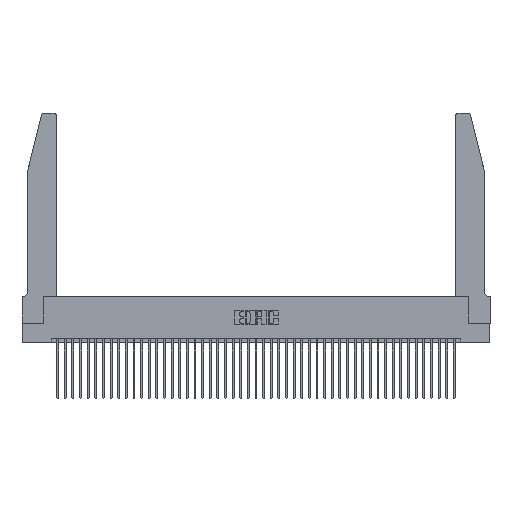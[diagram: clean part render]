
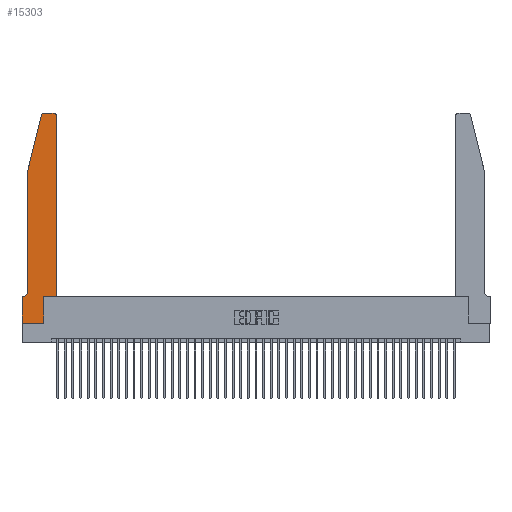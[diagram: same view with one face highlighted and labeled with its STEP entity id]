
A CAD part, top view. The second image highlights one B-rep face of the part: STEP entity #15303.
In plain terms, the highlighted planar face has unit normal (0, 0, 1).
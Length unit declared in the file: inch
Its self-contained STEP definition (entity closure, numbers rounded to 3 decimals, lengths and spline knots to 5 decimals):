
#76 = CARTESIAN_POINT ( 'NONE',  ( 0.0755, 0.35, 0.37 ) ) ;
#710 = DIRECTION ( 'NONE',  ( 1., 0., 0. ) ) ;
#795 = VERTEX_POINT ( 'NONE', #36567 ) ;
#1009 = CARTESIAN_POINT ( 'NONE',  ( 0., 0., 0.37 ) ) ;
#1309 = EDGE_CURVE ( 'NONE', #44725, #22038, #30585, .T. ) ;
#1569 = LINE ( 'NONE', #36733, #19284 ) ;
#1660 = DIRECTION ( 'NONE',  ( 0., 0., 1. ) ) ;
#2076 = VECTOR ( 'NONE', #38188, 39.37008 ) ;
#2180 = CIRCLE ( 'NONE', #6765, 0.07 ) ;
#2772 = VECTOR ( 'NONE', #710, 39.37008 ) ;
#3367 = DIRECTION ( 'NONE',  ( 0., 1., 0. ) ) ;
#3977 = AXIS2_PLACEMENT_3D ( 'NONE', #22750, #1660, #26181 ) ;
#4486 = EDGE_CURVE ( 'NONE', #9154, #10186, #36277, .T. ) ;
#6324 = DIRECTION ( 'NONE',  ( 0., 0., 1. ) ) ;
#6765 = AXIS2_PLACEMENT_3D ( 'NONE', #12347, #36340, #15891 ) ;
#7992 = ORIENTED_EDGE ( 'NONE', *, *, #33383, .T. ) ;
#8782 = EDGE_LOOP ( 'NONE', ( #35161, #17782, #32052, #16787, #7992, #31920, #22586, #39073, #15996, #11675, #17473, #20082 ) ) ;
#9097 = LINE ( 'NONE', #11024, #27553 ) ;
#9154 = VERTEX_POINT ( 'NONE', #36543 ) ;
#9280 = FACE_OUTER_BOUND ( 'NONE', #8782, .T. ) ;
#9546 = CARTESIAN_POINT ( 'NONE',  ( 0.0755, 2., 0.37 ) ) ;
#10186 = VERTEX_POINT ( 'NONE', #36451 ) ;
#11024 = CARTESIAN_POINT ( 'NONE',  ( 0.4505, 0.35, 0.37 ) ) ;
#11675 = ORIENTED_EDGE ( 'NONE', *, *, #24936, .T. ) ;
#12158 = EDGE_CURVE ( 'NONE', #10186, #16158, #44568, .T. ) ;
#12252 = CARTESIAN_POINT ( 'NONE',  ( 0.0755, 0.42, 0.37 ) ) ;
#12347 = CARTESIAN_POINT ( 'NONE',  ( 0.0055, 0.42, 0.37 ) ) ;
#13258 = LINE ( 'NONE', #28076, #21433 ) ;
#13936 = CARTESIAN_POINT ( 'NONE',  ( 0.2865, 0.35, 0.37 ) ) ;
#14322 = EDGE_CURVE ( 'NONE', #16159, #38533, #41130, .T. ) ;
#14345 = DIRECTION ( 'NONE',  ( 0., -1., 0. ) ) ;
#14538 = DIRECTION ( 'NONE',  ( 1., 0., 0. ) ) ;
#14761 = VERTEX_POINT ( 'NONE', #37540 ) ;
#15277 = DIRECTION ( 'NONE',  ( -0.239, -0.971, 0. ) ) ;
#15303 = ADVANCED_FACE ( 'NONE', ( #9280 ), #23843, .T. ) ;
#15891 = DIRECTION ( 'NONE',  ( -1., 0., 0. ) ) ;
#15937 = CARTESIAN_POINT ( 'NONE',  ( 0.0055, 0.35, 0.37 ) ) ;
#15996 = ORIENTED_EDGE ( 'NONE', *, *, #26676, .T. ) ;
#16158 = VERTEX_POINT ( 'NONE', #12252 ) ;
#16159 = VERTEX_POINT ( 'NONE', #15937 ) ;
#16787 = ORIENTED_EDGE ( 'NONE', *, *, #12158, .T. ) ;
#17473 = ORIENTED_EDGE ( 'NONE', *, *, #34103, .T. ) ;
#17782 = ORIENTED_EDGE ( 'NONE', *, *, #41490, .T. ) ;
#18174 = VECTOR ( 'NONE', #15277, 39.37008 ) ;
#19284 = VECTOR ( 'NONE', #40191, 39.37008 ) ;
#19387 = VERTEX_POINT ( 'NONE', #30235 ) ;
#20082 = ORIENTED_EDGE ( 'NONE', *, *, #31767, .T. ) ;
#20347 = CARTESIAN_POINT ( 'NONE',  ( 0.284, 2.72, 0.37 ) ) ;
#20458 = CARTESIAN_POINT ( 'NONE',  ( 0., 0., 0.37 ) ) ;
#20937 = EDGE_CURVE ( 'NONE', #38533, #44725, #39913, .T. ) ;
#21433 = VECTOR ( 'NONE', #34886, 39.37008 ) ;
#21814 = VECTOR ( 'NONE', #14345, 39.37008 ) ;
#22038 = VERTEX_POINT ( 'NONE', #27486 ) ;
#22586 = ORIENTED_EDGE ( 'NONE', *, *, #20937, .T. ) ;
#22750 = CARTESIAN_POINT ( 'NONE',  ( 0.4205, 2.72, 0.37 ) ) ;
#23774 = DIRECTION ( 'NONE',  ( 1., 0., 0. ) ) ;
#23843 = PLANE ( 'NONE',  #43394 ) ;
#24936 = EDGE_CURVE ( 'NONE', #40113, #19387, #9097, .T. ) ;
#26181 = DIRECTION ( 'NONE',  ( 1., 0., 0. ) ) ;
#26426 = VECTOR ( 'NONE', #37047, 39.37008 ) ;
#26676 = EDGE_CURVE ( 'NONE', #22038, #40113, #41310, .T. ) ;
#27154 = CARTESIAN_POINT ( 'NONE',  ( 0., 0.35, 0.37 ) ) ;
#27486 = CARTESIAN_POINT ( 'NONE',  ( 0.2865, 0., 0.37 ) ) ;
#27553 = VECTOR ( 'NONE', #14538, 39.37008 ) ;
#28076 = CARTESIAN_POINT ( 'NONE',  ( 0.2605, 2.75, 0.37 ) ) ;
#28304 = EDGE_CURVE ( 'NONE', #795, #14761, #13258, .T. ) ;
#28943 = CARTESIAN_POINT ( 'NONE',  ( 0.0755, 2., 0.37 ) ) ;
#30235 = CARTESIAN_POINT ( 'NONE',  ( 0.4505, 0.35, 0.37 ) ) ;
#30550 = DIRECTION ( 'NONE',  ( 1., 0., 0. ) ) ;
#30585 = LINE ( 'NONE', #1009, #2772 ) ;
#31767 = EDGE_CURVE ( 'NONE', #40876, #795, #31797, .T. ) ;
#31797 = CIRCLE ( 'NONE', #3977, 0.03 ) ;
#31920 = ORIENTED_EDGE ( 'NONE', *, *, #14322, .T. ) ;
#32052 = ORIENTED_EDGE ( 'NONE', *, *, #4486, .T. ) ;
#33383 = EDGE_CURVE ( 'NONE', #16158, #16159, #2180, .T. ) ;
#33966 = AXIS2_PLACEMENT_3D ( 'NONE', #20347, #44177, #23774 ) ;
#34103 = EDGE_CURVE ( 'NONE', #19387, #40876, #1569, .T. ) ;
#34222 = CARTESIAN_POINT ( 'NONE',  ( 0.4505, 2.72, 0.37 ) ) ;
#34863 = CARTESIAN_POINT ( 'NONE',  ( 0., 0., 0.37 ) ) ;
#34886 = DIRECTION ( 'NONE',  ( -1., 0., 0. ) ) ;
#35161 = ORIENTED_EDGE ( 'NONE', *, *, #28304, .T. ) ;
#36277 = LINE ( 'NONE', #28943, #18174 ) ;
#36340 = DIRECTION ( 'NONE',  ( 0., 0., -1. ) ) ;
#36451 = CARTESIAN_POINT ( 'NONE',  ( 0.0755, 2., 0.37 ) ) ;
#36543 = CARTESIAN_POINT ( 'NONE',  ( 0.25487, 2.72718, 0.37 ) ) ;
#36567 = CARTESIAN_POINT ( 'NONE',  ( 0.4205, 2.75, 0.37 ) ) ;
#36733 = CARTESIAN_POINT ( 'NONE',  ( 0.4505, 0.35, 0.37 ) ) ;
#37047 = DIRECTION ( 'NONE',  ( 0., -1., 0. ) ) ;
#37140 = CARTESIAN_POINT ( 'NONE',  ( 0., 0.35, 0.37 ) ) ;
#37540 = CARTESIAN_POINT ( 'NONE',  ( 0.284, 2.75, 0.37 ) ) ;
#38188 = DIRECTION ( 'NONE',  ( -1., 0., 0. ) ) ;
#38533 = VERTEX_POINT ( 'NONE', #37140 ) ;
#39073 = ORIENTED_EDGE ( 'NONE', *, *, #1309, .T. ) ;
#39913 = LINE ( 'NONE', #34863, #21814 ) ;
#40113 = VERTEX_POINT ( 'NONE', #40537 ) ;
#40191 = DIRECTION ( 'NONE',  ( 0., 1., 0. ) ) ;
#40216 = VECTOR ( 'NONE', #3367, 39.37008 ) ;
#40537 = CARTESIAN_POINT ( 'NONE',  ( 0.2865, 0.35, 0.37 ) ) ;
#40876 = VERTEX_POINT ( 'NONE', #34222 ) ;
#41130 = LINE ( 'NONE', #76, #2076 ) ;
#41310 = LINE ( 'NONE', #13936, #40216 ) ;
#41339 = CIRCLE ( 'NONE', #33966, 0.03 ) ;
#41490 = EDGE_CURVE ( 'NONE', #14761, #9154, #41339, .T. ) ;
#43394 = AXIS2_PLACEMENT_3D ( 'NONE', #27154, #6324, #30550 ) ;
#44177 = DIRECTION ( 'NONE',  ( 0., 0., 1. ) ) ;
#44568 = LINE ( 'NONE', #9546, #26426 ) ;
#44725 = VERTEX_POINT ( 'NONE', #20458 ) ;
